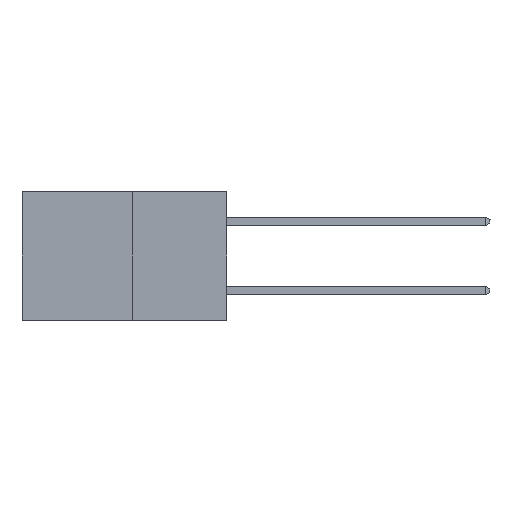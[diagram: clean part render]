
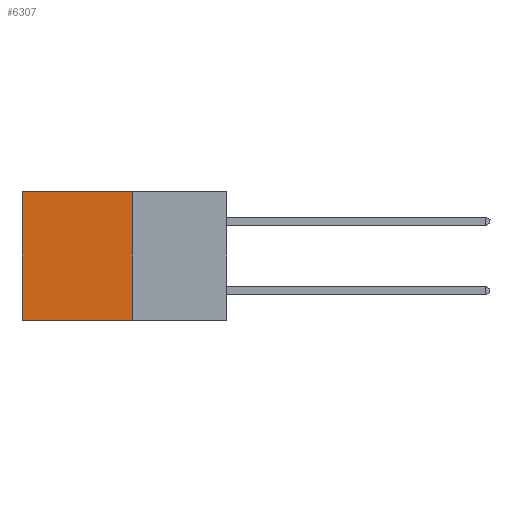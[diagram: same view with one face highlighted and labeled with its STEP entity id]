
A CAD part, left-side view. The second image highlights one B-rep face of the part: STEP entity #6307.
In plain terms, the highlighted planar face has unit normal (-1, 0, 0).
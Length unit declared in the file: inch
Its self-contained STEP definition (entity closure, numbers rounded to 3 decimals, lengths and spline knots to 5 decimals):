
#107 = CARTESIAN_POINT ( 'NONE',  ( 0.277, 0.27, 0. ) ) ;
#1074 = ORIENTED_EDGE ( 'NONE', *, *, #7503, .F. ) ;
#1077 = EDGE_CURVE ( 'NONE', #6506, #8802, #4142, .T. ) ;
#1448 = DIRECTION ( 'NONE',  ( 0., 1., 0. ) ) ;
#2794 = VERTEX_POINT ( 'NONE', #107 ) ;
#3237 = CARTESIAN_POINT ( 'NONE',  ( 0.277, 0.27, -0.37 ) ) ;
#3474 = CARTESIAN_POINT ( 'NONE',  ( 0.277, 0.59, -0.37 ) ) ;
#3529 = VECTOR ( 'NONE', #5398, 39.37008 ) ;
#3870 = EDGE_LOOP ( 'NONE', ( #9340, #5197, #1074, #7833 ) ) ;
#4142 = LINE ( 'NONE', #4155, #8785 ) ;
#4155 = CARTESIAN_POINT ( 'NONE',  ( 0.277, 0.59, -0.37 ) ) ;
#5046 = DIRECTION ( 'NONE',  ( 1., 0., 0. ) ) ;
#5093 = EDGE_CURVE ( 'NONE', #2794, #6506, #7793, .T. ) ;
#5197 = ORIENTED_EDGE ( 'NONE', *, *, #7358, .F. ) ;
#5287 = VECTOR ( 'NONE', #7724, 39.37008 ) ;
#5398 = DIRECTION ( 'NONE',  ( 0., 0., -1. ) ) ;
#5738 = VERTEX_POINT ( 'NONE', #6378 ) ;
#5942 = LINE ( 'NONE', #10882, #3529 ) ;
#6147 = FACE_OUTER_BOUND ( 'NONE', #3870, .T. ) ;
#6189 = DIRECTION ( 'NONE',  ( 0., 0., -1. ) ) ;
#6307 = ADVANCED_FACE ( 'NONE', ( #6147 ), #10558, .F. ) ;
#6378 = CARTESIAN_POINT ( 'NONE',  ( 0.277, 0.27, -0.37 ) ) ;
#6506 = VERTEX_POINT ( 'NONE', #9272 ) ;
#7358 = EDGE_CURVE ( 'NONE', #5738, #8802, #8307, .T. ) ;
#7503 = EDGE_CURVE ( 'NONE', #2794, #5738, #5942, .T. ) ;
#7724 = DIRECTION ( 'NONE',  ( 0., 1., 0. ) ) ;
#7793 = LINE ( 'NONE', #8023, #5287 ) ;
#7833 = ORIENTED_EDGE ( 'NONE', *, *, #5093, .T. ) ;
#8023 = CARTESIAN_POINT ( 'NONE',  ( 0.277, 0.27, 0. ) ) ;
#8307 = LINE ( 'NONE', #8832, #10952 ) ;
#8785 = VECTOR ( 'NONE', #6189, 39.37008 ) ;
#8802 = VERTEX_POINT ( 'NONE', #3474 ) ;
#8832 = CARTESIAN_POINT ( 'NONE',  ( 0.277, 0.27, -0.37 ) ) ;
#9272 = CARTESIAN_POINT ( 'NONE',  ( 0.277, 0.59, 0. ) ) ;
#9340 = ORIENTED_EDGE ( 'NONE', *, *, #1077, .T. ) ;
#10558 = PLANE ( 'NONE',  #11576 ) ;
#10882 = CARTESIAN_POINT ( 'NONE',  ( 0.277, 0.27, -0.37 ) ) ;
#10952 = VECTOR ( 'NONE', #1448, 39.37008 ) ;
#11391 = DIRECTION ( 'NONE',  ( 0., 0., -1. ) ) ;
#11576 = AXIS2_PLACEMENT_3D ( 'NONE', #3237, #5046, #11391 ) ;
